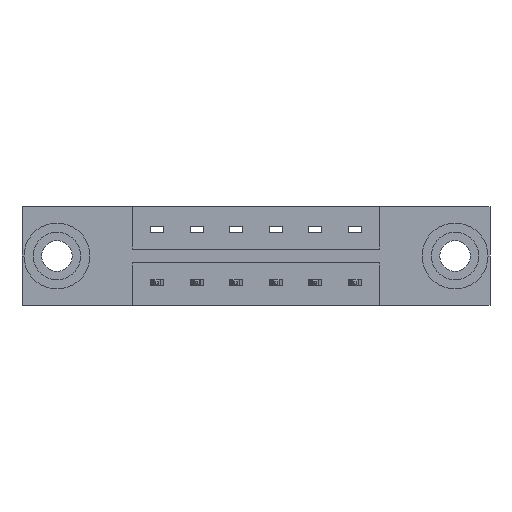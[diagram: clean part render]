
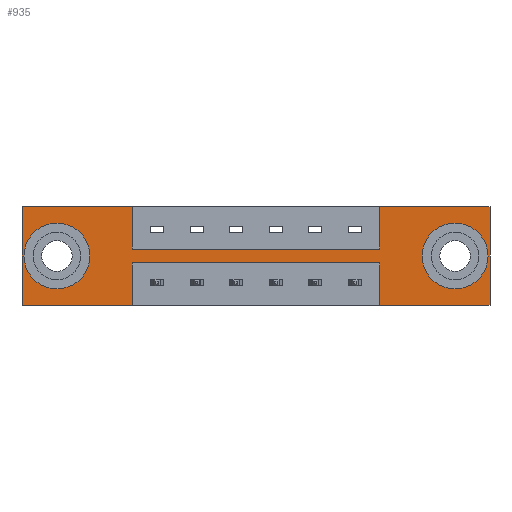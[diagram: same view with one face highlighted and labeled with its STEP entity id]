
A CAD part, front view. The second image highlights one B-rep face of the part: STEP entity #935.
In plain terms, the highlighted planar face has unit normal (0, -1, 0).
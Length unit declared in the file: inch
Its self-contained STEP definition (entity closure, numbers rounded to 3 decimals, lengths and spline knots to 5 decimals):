
#250 = EDGE_CURVE ( 'NONE', #8453, #3870, #1246, .T. ) ;
#335 = DIRECTION ( 'NONE',  ( 0., 0., 1. ) ) ;
#375 = LINE ( 'NONE', #4184, #8091 ) ;
#402 = AXIS2_PLACEMENT_3D ( 'NONE', #8232, #3297, #6066 ) ;
#417 = CARTESIAN_POINT ( 'NONE',  ( 0., 0., 0. ) ) ;
#491 = VECTOR ( 'NONE', #335, 39.37008 ) ;
#703 = ORIENTED_EDGE ( 'NONE', *, *, #5585, .F. ) ;
#795 = CIRCLE ( 'NONE', #2516, 0.078 ) ;
#836 = ORIENTED_EDGE ( 'NONE', *, *, #4515, .F. ) ;
#935 = ADVANCED_FACE ( 'NONE', ( #6586, #1759, #8186 ), #3365, .T. ) ;
#985 = LINE ( 'NONE', #4383, #4027 ) ;
#1061 = CARTESIAN_POINT ( 'NONE',  ( 1.775, 0., -0.375 ) ) ;
#1246 = LINE ( 'NONE', #1670, #491 ) ;
#1396 = EDGE_LOOP ( 'NONE', ( #4115, #6530 ) ) ;
#1522 = VECTOR ( 'NONE', #4769, 39.37008 ) ;
#1536 = CARTESIAN_POINT ( 'NONE',  ( 1.775, 0., 0. ) ) ;
#1562 = EDGE_CURVE ( 'NONE', #7264, #1915, #795, .T. ) ;
#1607 = AXIS2_PLACEMENT_3D ( 'NONE', #3512, #8371, #5760 ) ;
#1670 = CARTESIAN_POINT ( 'NONE',  ( 1.3575, 0., -0.214 ) ) ;
#1759 = FACE_BOUND ( 'NONE', #1396, .T. ) ;
#1903 = DIRECTION ( 'NONE',  ( -1., 0., 0. ) ) ;
#1915 = VERTEX_POINT ( 'NONE', #2389 ) ;
#1918 = VERTEX_POINT ( 'NONE', #4988 ) ;
#1946 = LINE ( 'NONE', #1536, #7519 ) ;
#1955 = CARTESIAN_POINT ( 'NONE',  ( 1.6425, 0., -0.1875 ) ) ;
#1972 = LINE ( 'NONE', #5953, #7987 ) ;
#2088 = EDGE_CURVE ( 'NONE', #8722, #6424, #3501, .T. ) ;
#2089 = DIRECTION ( 'NONE',  ( -1., 0., 0. ) ) ;
#2121 = CIRCLE ( 'NONE', #1607, 0.078 ) ;
#2129 = VECTOR ( 'NONE', #6921, 39.37008 ) ;
#2193 = CARTESIAN_POINT ( 'NONE',  ( 1.6425, 0., -0.1095 ) ) ;
#2203 = CARTESIAN_POINT ( 'NONE',  ( 1.3575, 0., -0.375 ) ) ;
#2308 = DIRECTION ( 'NONE',  ( 1., 0., 0. ) ) ;
#2319 = ORIENTED_EDGE ( 'NONE', *, *, #7537, .F. ) ;
#2335 = VECTOR ( 'NONE', #7646, 39.37008 ) ;
#2389 = CARTESIAN_POINT ( 'NONE',  ( 1.6425, 0., -0.2655 ) ) ;
#2408 = VERTEX_POINT ( 'NONE', #4648 ) ;
#2516 = AXIS2_PLACEMENT_3D ( 'NONE', #8527, #3755, #4484 ) ;
#2570 = CARTESIAN_POINT ( 'NONE',  ( 1.3575, 0., -0.161 ) ) ;
#2587 = CARTESIAN_POINT ( 'NONE',  ( 0.4175, 0., -0.161 ) ) ;
#2611 = DIRECTION ( 'NONE',  ( 0., 0., -1. ) ) ;
#2763 = LINE ( 'NONE', #4248, #2335 ) ;
#2797 = EDGE_CURVE ( 'NONE', #3551, #4345, #1946, .T. ) ;
#3179 = VERTEX_POINT ( 'NONE', #7658 ) ;
#3195 = VERTEX_POINT ( 'NONE', #4196 ) ;
#3200 = ORIENTED_EDGE ( 'NONE', *, *, #5120, .F. ) ;
#3209 = EDGE_CURVE ( 'NONE', #6292, #4333, #7207, .T. ) ;
#3297 = DIRECTION ( 'NONE',  ( 0., -1., 0. ) ) ;
#3339 = LINE ( 'NONE', #6782, #8664 ) ;
#3365 = PLANE ( 'NONE',  #402 ) ;
#3498 = EDGE_CURVE ( 'NONE', #4345, #8453, #985, .T. ) ;
#3501 = CIRCLE ( 'NONE', #6457, 0.078 ) ;
#3512 = CARTESIAN_POINT ( 'NONE',  ( 0.1325, 0., -0.1875 ) ) ;
#3551 = VERTEX_POINT ( 'NONE', #5660 ) ;
#3656 = DIRECTION ( 'NONE',  ( -1., 0., 0. ) ) ;
#3755 = DIRECTION ( 'NONE',  ( 0., 1., 0. ) ) ;
#3803 = VECTOR ( 'NONE', #7333, 39.37008 ) ;
#3870 = VERTEX_POINT ( 'NONE', #6546 ) ;
#3941 = DIRECTION ( 'NONE',  ( 0., 0., 1. ) ) ;
#4011 = ORIENTED_EDGE ( 'NONE', *, *, #8170, .T. ) ;
#4027 = VECTOR ( 'NONE', #3656, 39.37008 ) ;
#4092 = CARTESIAN_POINT ( 'NONE',  ( 0., 0., 0. ) ) ;
#4115 = ORIENTED_EDGE ( 'NONE', *, *, #2088, .T. ) ;
#4184 = CARTESIAN_POINT ( 'NONE',  ( 0.4175, 0., -0.214 ) ) ;
#4196 = CARTESIAN_POINT ( 'NONE',  ( 0., 0., -0.375 ) ) ;
#4225 = LINE ( 'NONE', #4092, #2129 ) ;
#4248 = CARTESIAN_POINT ( 'NONE',  ( 0.4175, 0., -0.161 ) ) ;
#4333 = VERTEX_POINT ( 'NONE', #6639 ) ;
#4345 = VERTEX_POINT ( 'NONE', #1061 ) ;
#4383 = CARTESIAN_POINT ( 'NONE',  ( 0., 0., -0.375 ) ) ;
#4484 = DIRECTION ( 'NONE',  ( 0., 0., -1. ) ) ;
#4515 = EDGE_CURVE ( 'NONE', #3179, #3195, #3339, .T. ) ;
#4564 = EDGE_LOOP ( 'NONE', ( #4651, #4011 ) ) ;
#4648 = CARTESIAN_POINT ( 'NONE',  ( 0.4175, 0., 0. ) ) ;
#4651 = ORIENTED_EDGE ( 'NONE', *, *, #1562, .T. ) ;
#4769 = DIRECTION ( 'NONE',  ( 0., 0., 1. ) ) ;
#4873 = ORIENTED_EDGE ( 'NONE', *, *, #5160, .F. ) ;
#4917 = LINE ( 'NONE', #8014, #5462 ) ;
#4981 = CARTESIAN_POINT ( 'NONE',  ( 0.1325, 0., -0.2655 ) ) ;
#4988 = CARTESIAN_POINT ( 'NONE',  ( 0.4175, 0., -0.214 ) ) ;
#5120 = EDGE_CURVE ( 'NONE', #4333, #3551, #4225, .T. ) ;
#5160 = EDGE_CURVE ( 'NONE', #2408, #8215, #2763, .T. ) ;
#5240 = DIRECTION ( 'NONE',  ( 1., 0., 0. ) ) ;
#5303 = ORIENTED_EDGE ( 'NONE', *, *, #2797, .F. ) ;
#5325 = AXIS2_PLACEMENT_3D ( 'NONE', #1955, #8810, #2611 ) ;
#5345 = ORIENTED_EDGE ( 'NONE', *, *, #8755, .F. ) ;
#5443 = EDGE_CURVE ( 'NONE', #6424, #8722, #2121, .T. ) ;
#5462 = VECTOR ( 'NONE', #5240, 39.37008 ) ;
#5526 = ORIENTED_EDGE ( 'NONE', *, *, #3498, .F. ) ;
#5585 = EDGE_CURVE ( 'NONE', #3195, #7534, #8270, .T. ) ;
#5660 = CARTESIAN_POINT ( 'NONE',  ( 1.775, 0., 0. ) ) ;
#5713 = ORIENTED_EDGE ( 'NONE', *, *, #3209, .F. ) ;
#5724 = EDGE_CURVE ( 'NONE', #3870, #1918, #375, .T. ) ;
#5760 = DIRECTION ( 'NONE',  ( 0., 0., 1. ) ) ;
#5924 = EDGE_CURVE ( 'NONE', #7534, #2408, #1972, .T. ) ;
#5940 = CARTESIAN_POINT ( 'NONE',  ( 0.4175, 0., -0.214 ) ) ;
#5953 = CARTESIAN_POINT ( 'NONE',  ( 0., 0., 0. ) ) ;
#6066 = DIRECTION ( 'NONE',  ( 0., 0., -1. ) ) ;
#6122 = VECTOR ( 'NONE', #7492, 39.37008 ) ;
#6129 = CARTESIAN_POINT ( 'NONE',  ( 0., 0., 0. ) ) ;
#6292 = VERTEX_POINT ( 'NONE', #6531 ) ;
#6387 = ORIENTED_EDGE ( 'NONE', *, *, #250, .F. ) ;
#6424 = VERTEX_POINT ( 'NONE', #4981 ) ;
#6457 = AXIS2_PLACEMENT_3D ( 'NONE', #8097, #8046, #3941 ) ;
#6530 = ORIENTED_EDGE ( 'NONE', *, *, #5443, .T. ) ;
#6531 = CARTESIAN_POINT ( 'NONE',  ( 1.3575, 0., -0.161 ) ) ;
#6546 = CARTESIAN_POINT ( 'NONE',  ( 1.3575, 0., -0.214 ) ) ;
#6586 = FACE_BOUND ( 'NONE', #4564, .T. ) ;
#6639 = CARTESIAN_POINT ( 'NONE',  ( 1.3575, 0., 0. ) ) ;
#6782 = CARTESIAN_POINT ( 'NONE',  ( 0., 0., -0.375 ) ) ;
#6866 = LINE ( 'NONE', #5940, #3803 ) ;
#6921 = DIRECTION ( 'NONE',  ( 1., 0., 0. ) ) ;
#7170 = ORIENTED_EDGE ( 'NONE', *, *, #5924, .F. ) ;
#7207 = LINE ( 'NONE', #2570, #1522 ) ;
#7264 = VERTEX_POINT ( 'NONE', #2193 ) ;
#7333 = DIRECTION ( 'NONE',  ( 0., 0., -1. ) ) ;
#7492 = DIRECTION ( 'NONE',  ( 0., 0., 1. ) ) ;
#7519 = VECTOR ( 'NONE', #8136, 39.37008 ) ;
#7534 = VERTEX_POINT ( 'NONE', #417 ) ;
#7537 = EDGE_CURVE ( 'NONE', #8215, #6292, #4917, .T. ) ;
#7646 = DIRECTION ( 'NONE',  ( 0., 0., -1. ) ) ;
#7658 = CARTESIAN_POINT ( 'NONE',  ( 0.4175, 0., -0.375 ) ) ;
#7987 = VECTOR ( 'NONE', #2308, 39.37008 ) ;
#8014 = CARTESIAN_POINT ( 'NONE',  ( 0.4175, 0., -0.161 ) ) ;
#8046 = DIRECTION ( 'NONE',  ( 0., 1., 0. ) ) ;
#8091 = VECTOR ( 'NONE', #2089, 39.37008 ) ;
#8097 = CARTESIAN_POINT ( 'NONE',  ( 0.1325, 0., -0.1875 ) ) ;
#8136 = DIRECTION ( 'NONE',  ( 0., 0., -1. ) ) ;
#8170 = EDGE_CURVE ( 'NONE', #1915, #7264, #8592, .T. ) ;
#8186 = FACE_OUTER_BOUND ( 'NONE', #8272, .T. ) ;
#8204 = ORIENTED_EDGE ( 'NONE', *, *, #5724, .F. ) ;
#8215 = VERTEX_POINT ( 'NONE', #2587 ) ;
#8232 = CARTESIAN_POINT ( 'NONE',  ( 0., 0., -0.375 ) ) ;
#8270 = LINE ( 'NONE', #6129, #6122 ) ;
#8272 = EDGE_LOOP ( 'NONE', ( #6387, #5526, #5303, #3200, #5713, #2319, #4873, #7170, #703, #836, #5345, #8204 ) ) ;
#8371 = DIRECTION ( 'NONE',  ( 0., 1., 0. ) ) ;
#8453 = VERTEX_POINT ( 'NONE', #2203 ) ;
#8527 = CARTESIAN_POINT ( 'NONE',  ( 1.6425, 0., -0.1875 ) ) ;
#8592 = CIRCLE ( 'NONE', #5325, 0.078 ) ;
#8664 = VECTOR ( 'NONE', #1903, 39.37008 ) ;
#8722 = VERTEX_POINT ( 'NONE', #8737 ) ;
#8737 = CARTESIAN_POINT ( 'NONE',  ( 0.1325, 0., -0.1095 ) ) ;
#8755 = EDGE_CURVE ( 'NONE', #1918, #3179, #6866, .T. ) ;
#8810 = DIRECTION ( 'NONE',  ( 0., 1., 0. ) ) ;
